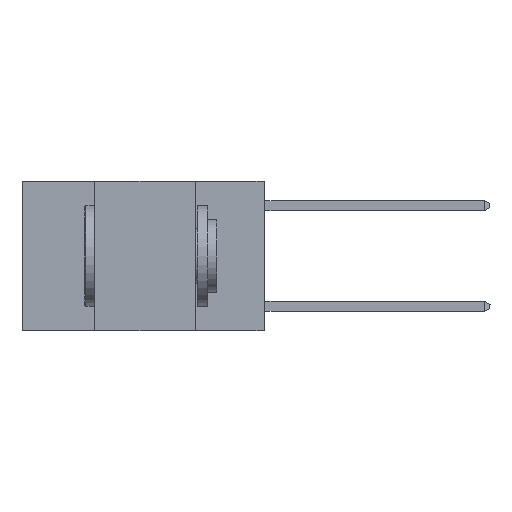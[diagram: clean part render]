
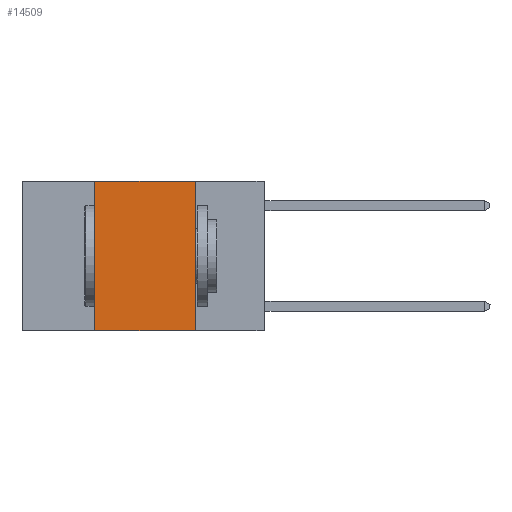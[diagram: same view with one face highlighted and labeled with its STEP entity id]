
A CAD part, left-side view. The second image highlights one B-rep face of the part: STEP entity #14509.
In plain terms, the highlighted planar face has unit normal (-1, 0, 0).
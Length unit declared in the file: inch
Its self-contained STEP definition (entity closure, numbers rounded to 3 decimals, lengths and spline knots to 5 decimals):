
#1655 = VERTEX_POINT ( 'NONE', #24397 ) ;
#2364 = LINE ( 'NONE', #6775, #8759 ) ;
#3060 = CARTESIAN_POINT ( 'NONE',  ( 0., 0.6, -0.37 ) ) ;
#3273 = VERTEX_POINT ( 'NONE', #8306 ) ;
#4518 = DIRECTION ( 'NONE',  ( 0., -1., 0. ) ) ;
#4738 = ORIENTED_EDGE ( 'NONE', *, *, #10650, .F. ) ;
#5233 = FACE_OUTER_BOUND ( 'NONE', #13298, .T. ) ;
#5775 = DIRECTION ( 'NONE',  ( 1., 0., 0. ) ) ;
#6070 = ORIENTED_EDGE ( 'NONE', *, *, #21294, .F. ) ;
#6718 = DIRECTION ( 'NONE',  ( 0., 0., 1. ) ) ;
#6775 = CARTESIAN_POINT ( 'NONE',  ( 0., 0.6, 0. ) ) ;
#7393 = DIRECTION ( 'NONE',  ( 0., -1., 0. ) ) ;
#7511 = CARTESIAN_POINT ( 'NONE',  ( 0., 0.42, -0.37 ) ) ;
#8306 = CARTESIAN_POINT ( 'NONE',  ( 0., 0.17, 0. ) ) ;
#8759 = VECTOR ( 'NONE', #4518, 39.37008 ) ;
#9913 = PLANE ( 'NONE',  #24839 ) ;
#10457 = ORIENTED_EDGE ( 'NONE', *, *, #22424, .F. ) ;
#10650 = EDGE_CURVE ( 'NONE', #3273, #1655, #25546, .T. ) ;
#10662 = DIRECTION ( 'NONE',  ( 0., 0., -1. ) ) ;
#12877 = LINE ( 'NONE', #26005, #23585 ) ;
#13298 = EDGE_LOOP ( 'NONE', ( #4738, #10457, #6070, #14510 ) ) ;
#13382 = LINE ( 'NONE', #3060, #24084 ) ;
#13553 = CARTESIAN_POINT ( 'NONE',  ( 0., 0.42, 0. ) ) ;
#14509 = ADVANCED_FACE ( 'NONE', ( #5233 ), #9913, .F. ) ;
#14510 = ORIENTED_EDGE ( 'NONE', *, *, #25409, .T. ) ;
#14911 = CARTESIAN_POINT ( 'NONE',  ( 0., 0.17, 0. ) ) ;
#15611 = VERTEX_POINT ( 'NONE', #13553 ) ;
#18669 = CARTESIAN_POINT ( 'NONE',  ( 0., 0.6, 0. ) ) ;
#19877 = VECTOR ( 'NONE', #10662, 39.37008 ) ;
#20794 = DIRECTION ( 'NONE',  ( 0., 0., -1. ) ) ;
#21294 = EDGE_CURVE ( 'NONE', #22679, #15611, #12877, .T. ) ;
#22424 = EDGE_CURVE ( 'NONE', #15611, #3273, #2364, .T. ) ;
#22679 = VERTEX_POINT ( 'NONE', #7511 ) ;
#23585 = VECTOR ( 'NONE', #6718, 39.37008 ) ;
#24084 = VECTOR ( 'NONE', #7393, 39.37008 ) ;
#24397 = CARTESIAN_POINT ( 'NONE',  ( 0., 0.17, -0.37 ) ) ;
#24839 = AXIS2_PLACEMENT_3D ( 'NONE', #18669, #5775, #20794 ) ;
#25409 = EDGE_CURVE ( 'NONE', #22679, #1655, #13382, .T. ) ;
#25546 = LINE ( 'NONE', #14911, #19877 ) ;
#26005 = CARTESIAN_POINT ( 'NONE',  ( 0., 0.42, 0. ) ) ;
